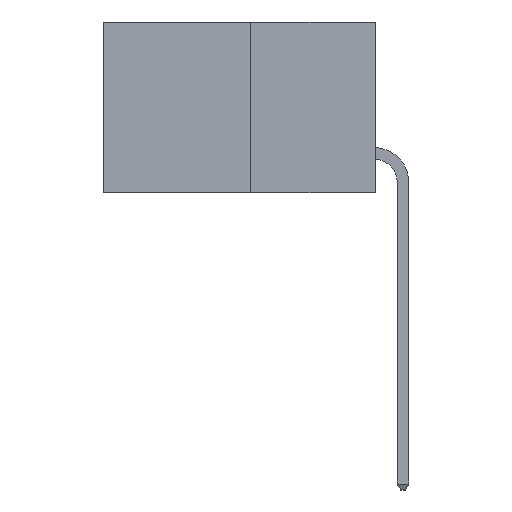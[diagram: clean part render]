
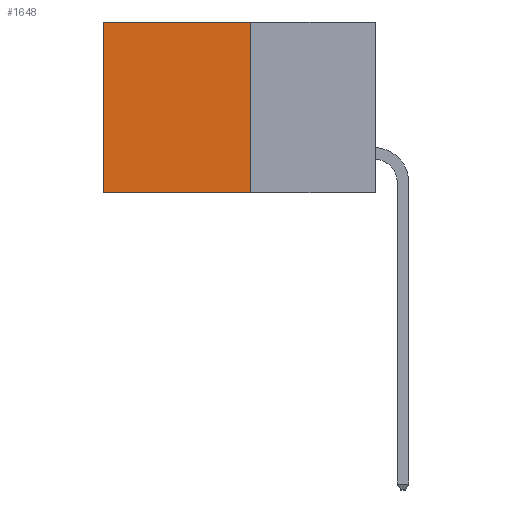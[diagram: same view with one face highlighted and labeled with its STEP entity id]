
A CAD part, left-side view. The second image highlights one B-rep face of the part: STEP entity #1648.
In plain terms, the highlighted planar face has unit normal (-1, 0, 0).
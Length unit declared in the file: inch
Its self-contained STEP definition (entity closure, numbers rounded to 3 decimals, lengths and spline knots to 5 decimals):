
#1353 = ORIENTED_EDGE ( 'NONE', *, *, #14439, .F. ) ;
#1648 = ADVANCED_FACE ( 'NONE', ( #12284 ), #5819, .F. ) ;
#1787 = AXIS2_PLACEMENT_3D ( 'NONE', #7559, #7480, #7476 ) ;
#1820 = CARTESIAN_POINT ( 'NONE',  ( 0.277, 0.27, -0.37 ) ) ;
#2373 = CARTESIAN_POINT ( 'NONE',  ( 0.277, 0.59, -0.37 ) ) ;
#2807 = DIRECTION ( 'NONE',  ( 0., 1., 0. ) ) ;
#5819 = PLANE ( 'NONE',  #1787 ) ;
#6064 = DIRECTION ( 'NONE',  ( 0., 0., -1. ) ) ;
#7365 = LINE ( 'NONE', #2373, #13446 ) ;
#7476 = DIRECTION ( 'NONE',  ( 0., 0., -1. ) ) ;
#7480 = DIRECTION ( 'NONE',  ( 1., 0., 0. ) ) ;
#7559 = CARTESIAN_POINT ( 'NONE',  ( 0.277, 0.27, -0.37 ) ) ;
#9345 = CARTESIAN_POINT ( 'NONE',  ( 0.277, 0.59, -0.37 ) ) ;
#9634 = VECTOR ( 'NONE', #18633, 39.37008 ) ;
#9843 = ORIENTED_EDGE ( 'NONE', *, *, #10311, .T. ) ;
#10311 = EDGE_CURVE ( 'NONE', #14769, #21827, #17412, .T. ) ;
#10684 = VECTOR ( 'NONE', #18479, 39.37008 ) ;
#11375 = ORIENTED_EDGE ( 'NONE', *, *, #23133, .F. ) ;
#11568 = VERTEX_POINT ( 'NONE', #9345 ) ;
#12284 = FACE_OUTER_BOUND ( 'NONE', #23674, .T. ) ;
#12469 = VECTOR ( 'NONE', #2807, 39.37008 ) ;
#13446 = VECTOR ( 'NONE', #6064, 39.37008 ) ;
#14439 = EDGE_CURVE ( 'NONE', #14769, #19157, #15600, .T. ) ;
#14769 = VERTEX_POINT ( 'NONE', #21381 ) ;
#14796 = CARTESIAN_POINT ( 'NONE',  ( 0.277, 0.59, 0. ) ) ;
#15600 = LINE ( 'NONE', #1820, #10684 ) ;
#15914 = CARTESIAN_POINT ( 'NONE',  ( 0.277, 0.27, 0. ) ) ;
#16794 = CARTESIAN_POINT ( 'NONE',  ( 0.277, 0.27, -0.37 ) ) ;
#16799 = CARTESIAN_POINT ( 'NONE',  ( 0.277, 0.27, -0.37 ) ) ;
#17412 = LINE ( 'NONE', #15914, #12469 ) ;
#18479 = DIRECTION ( 'NONE',  ( 0., 0., -1. ) ) ;
#18633 = DIRECTION ( 'NONE',  ( 0., 1., 0. ) ) ;
#19157 = VERTEX_POINT ( 'NONE', #16794 ) ;
#19332 = EDGE_CURVE ( 'NONE', #21827, #11568, #7365, .T. ) ;
#19434 = LINE ( 'NONE', #16799, #9634 ) ;
#21381 = CARTESIAN_POINT ( 'NONE',  ( 0.277, 0.27, 0. ) ) ;
#21827 = VERTEX_POINT ( 'NONE', #14796 ) ;
#22919 = ORIENTED_EDGE ( 'NONE', *, *, #19332, .T. ) ;
#23133 = EDGE_CURVE ( 'NONE', #19157, #11568, #19434, .T. ) ;
#23674 = EDGE_LOOP ( 'NONE', ( #22919, #11375, #1353, #9843 ) ) ;
